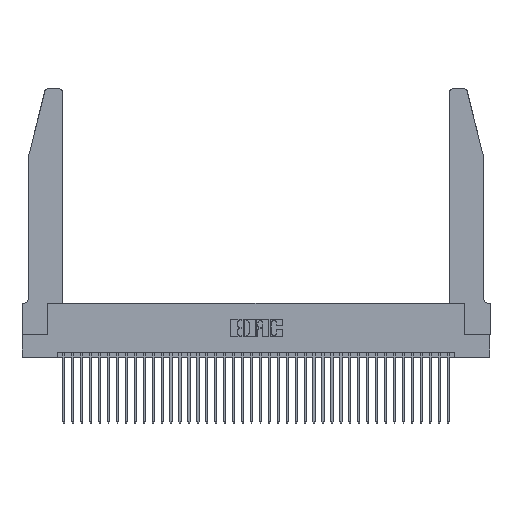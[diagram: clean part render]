
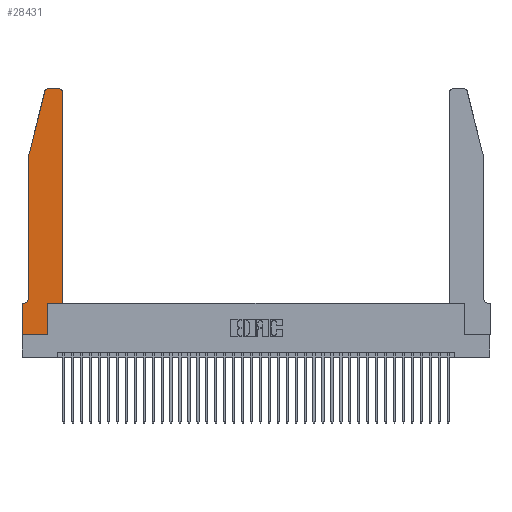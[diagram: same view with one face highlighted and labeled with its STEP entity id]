
A CAD part, top view. The second image highlights one B-rep face of the part: STEP entity #28431.
In plain terms, the highlighted planar face has unit normal (0, 0, 1).
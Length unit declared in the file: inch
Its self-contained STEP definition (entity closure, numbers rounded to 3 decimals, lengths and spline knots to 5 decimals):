
#224 = EDGE_CURVE ( 'NONE', #29891, #2892, #13376, .T. ) ;
#667 = CARTESIAN_POINT ( 'NONE',  ( 0.4505, 0.35, 0.37 ) ) ;
#727 = LINE ( 'NONE', #18603, #18625 ) ;
#1200 = VECTOR ( 'NONE', #37768, 39.37008 ) ;
#1596 = PLANE ( 'NONE',  #32120 ) ;
#1674 = ORIENTED_EDGE ( 'NONE', *, *, #16452, .T. ) ;
#2068 = DIRECTION ( 'NONE',  ( 1., 0., 0. ) ) ;
#2127 = VECTOR ( 'NONE', #15969, 39.37008 ) ;
#2576 = LINE ( 'NONE', #667, #2127 ) ;
#2687 = DIRECTION ( 'NONE',  ( -1., 0., 0. ) ) ;
#2892 = VERTEX_POINT ( 'NONE', #20717 ) ;
#4173 = VERTEX_POINT ( 'NONE', #35448 ) ;
#4774 = CARTESIAN_POINT ( 'NONE',  ( 0.2865, 0., 0.37 ) ) ;
#5202 = EDGE_CURVE ( 'NONE', #22852, #8527, #727, .T. ) ;
#5338 = CARTESIAN_POINT ( 'NONE',  ( 0.4505, 0.35, 0.37 ) ) ;
#5971 = CARTESIAN_POINT ( 'NONE',  ( 0., 0., 0.37 ) ) ;
#6291 = CARTESIAN_POINT ( 'NONE',  ( 0.284, 2.72, 0.37 ) ) ;
#6340 = ORIENTED_EDGE ( 'NONE', *, *, #35935, .T. ) ;
#6474 = ORIENTED_EDGE ( 'NONE', *, *, #19601, .T. ) ;
#7373 = FACE_OUTER_BOUND ( 'NONE', #20908, .T. ) ;
#7486 = VERTEX_POINT ( 'NONE', #33613 ) ;
#7542 = VECTOR ( 'NONE', #30701, 39.37008 ) ;
#7683 = ORIENTED_EDGE ( 'NONE', *, *, #36097, .T. ) ;
#8160 = VECTOR ( 'NONE', #17964, 39.37008 ) ;
#8347 = ORIENTED_EDGE ( 'NONE', *, *, #224, .T. ) ;
#8405 = VERTEX_POINT ( 'NONE', #4774 ) ;
#8527 = VERTEX_POINT ( 'NONE', #29966 ) ;
#9138 = CARTESIAN_POINT ( 'NONE',  ( 0.4505, 2.72, 0.37 ) ) ;
#9248 = ORIENTED_EDGE ( 'NONE', *, *, #34002, .T. ) ;
#10431 = VERTEX_POINT ( 'NONE', #27357 ) ;
#10446 = DIRECTION ( 'NONE',  ( 1., 0., 0. ) ) ;
#10654 = ORIENTED_EDGE ( 'NONE', *, *, #5202, .T. ) ;
#13376 = LINE ( 'NONE', #5971, #8160 ) ;
#14517 = EDGE_CURVE ( 'NONE', #10431, #18430, #16909, .T. ) ;
#15095 = LINE ( 'NONE', #36754, #7542 ) ;
#15705 = VECTOR ( 'NONE', #23273, 39.37008 ) ;
#15969 = DIRECTION ( 'NONE',  ( 0., 1., 0. ) ) ;
#16210 = ORIENTED_EDGE ( 'NONE', *, *, #38175, .T. ) ;
#16410 = ORIENTED_EDGE ( 'NONE', *, *, #17828, .T. ) ;
#16452 = EDGE_CURVE ( 'NONE', #2892, #8405, #31393, .T. ) ;
#16646 = LINE ( 'NONE', #16975, #15705 ) ;
#16909 = LINE ( 'NONE', #21971, #36721 ) ;
#16975 = CARTESIAN_POINT ( 'NONE',  ( 0.4505, 0.35, 0.37 ) ) ;
#17558 = EDGE_CURVE ( 'NONE', #18430, #4173, #30797, .T. ) ;
#17794 = LINE ( 'NONE', #25690, #23898 ) ;
#17828 = EDGE_CURVE ( 'NONE', #7486, #22150, #16646, .T. ) ;
#17964 = DIRECTION ( 'NONE',  ( 0., -1., 0. ) ) ;
#18154 = DIRECTION ( 'NONE',  ( 1., 0., 0. ) ) ;
#18430 = VERTEX_POINT ( 'NONE', #21197 ) ;
#18603 = CARTESIAN_POINT ( 'NONE',  ( 0.2605, 2.75, 0.37 ) ) ;
#18625 = VECTOR ( 'NONE', #21612, 39.37008 ) ;
#19601 = EDGE_CURVE ( 'NONE', #4173, #22254, #33695, .T. ) ;
#20607 = CARTESIAN_POINT ( 'NONE',  ( 0.0055, 0.42, 0.37 ) ) ;
#20717 = CARTESIAN_POINT ( 'NONE',  ( 0., 0., 0.37 ) ) ;
#20908 = EDGE_LOOP ( 'NONE', ( #10654, #6340, #33339, #28059, #6474, #20993, #8347, #1674, #7683, #16410, #9248, #16210 ) ) ;
#20993 = ORIENTED_EDGE ( 'NONE', *, *, #35702, .T. ) ;
#21197 = CARTESIAN_POINT ( 'NONE',  ( 0.0755, 2., 0.37 ) ) ;
#21612 = DIRECTION ( 'NONE',  ( -1., 0., 0. ) ) ;
#21971 = CARTESIAN_POINT ( 'NONE',  ( 0.0755, 2., 0.37 ) ) ;
#22077 = CARTESIAN_POINT ( 'NONE',  ( 0.0755, 2., 0.37 ) ) ;
#22150 = VERTEX_POINT ( 'NONE', #5338 ) ;
#22254 = VERTEX_POINT ( 'NONE', #30280 ) ;
#22585 = CARTESIAN_POINT ( 'NONE',  ( 0., 0., 0.37 ) ) ;
#22828 = CARTESIAN_POINT ( 'NONE',  ( 0., 0.35, 0.37 ) ) ;
#22852 = VERTEX_POINT ( 'NONE', #29315 ) ;
#23273 = DIRECTION ( 'NONE',  ( 1., 0., 0. ) ) ;
#23898 = VECTOR ( 'NONE', #28742, 39.37008 ) ;
#24985 = DIRECTION ( 'NONE',  ( 0., -1., 0. ) ) ;
#25690 = CARTESIAN_POINT ( 'NONE',  ( 0.0755, 0.35, 0.37 ) ) ;
#26410 = CIRCLE ( 'NONE', #27653, 0.03 ) ;
#26876 = VERTEX_POINT ( 'NONE', #9138 ) ;
#27357 = CARTESIAN_POINT ( 'NONE',  ( 0.25487, 2.72718, 0.37 ) ) ;
#27653 = AXIS2_PLACEMENT_3D ( 'NONE', #6291, #33208, #18154 ) ;
#27711 = AXIS2_PLACEMENT_3D ( 'NONE', #37686, #38213, #2068 ) ;
#28059 = ORIENTED_EDGE ( 'NONE', *, *, #17558, .T. ) ;
#28195 = DIRECTION ( 'NONE',  ( -0.239, -0.971, 0. ) ) ;
#28431 = ADVANCED_FACE ( 'NONE', ( #7373 ), #1596, .T. ) ;
#28493 = DIRECTION ( 'NONE',  ( 0., 0., 1. ) ) ;
#28742 = DIRECTION ( 'NONE',  ( -1., 0., 0. ) ) ;
#29315 = CARTESIAN_POINT ( 'NONE',  ( 0.4205, 2.75, 0.37 ) ) ;
#29629 = CIRCLE ( 'NONE', #27711, 0.03 ) ;
#29891 = VERTEX_POINT ( 'NONE', #22828 ) ;
#29966 = CARTESIAN_POINT ( 'NONE',  ( 0.284, 2.75, 0.37 ) ) ;
#30280 = CARTESIAN_POINT ( 'NONE',  ( 0.0055, 0.35, 0.37 ) ) ;
#30701 = DIRECTION ( 'NONE',  ( 0., 1., 0. ) ) ;
#30797 = LINE ( 'NONE', #22077, #38807 ) ;
#31393 = LINE ( 'NONE', #22585, #1200 ) ;
#32120 = AXIS2_PLACEMENT_3D ( 'NONE', #37730, #28493, #10446 ) ;
#33208 = DIRECTION ( 'NONE',  ( 0., 0., 1. ) ) ;
#33339 = ORIENTED_EDGE ( 'NONE', *, *, #14517, .T. ) ;
#33613 = CARTESIAN_POINT ( 'NONE',  ( 0.2865, 0.35, 0.37 ) ) ;
#33695 = CIRCLE ( 'NONE', #37466, 0.07 ) ;
#34002 = EDGE_CURVE ( 'NONE', #22150, #26876, #2576, .T. ) ;
#35448 = CARTESIAN_POINT ( 'NONE',  ( 0.0755, 0.42, 0.37 ) ) ;
#35702 = EDGE_CURVE ( 'NONE', #22254, #29891, #17794, .T. ) ;
#35824 = DIRECTION ( 'NONE',  ( 0., 0., -1. ) ) ;
#35935 = EDGE_CURVE ( 'NONE', #8527, #10431, #26410, .T. ) ;
#36097 = EDGE_CURVE ( 'NONE', #8405, #7486, #15095, .T. ) ;
#36721 = VECTOR ( 'NONE', #28195, 39.37008 ) ;
#36754 = CARTESIAN_POINT ( 'NONE',  ( 0.2865, 0.35, 0.37 ) ) ;
#37466 = AXIS2_PLACEMENT_3D ( 'NONE', #20607, #35824, #2687 ) ;
#37686 = CARTESIAN_POINT ( 'NONE',  ( 0.4205, 2.72, 0.37 ) ) ;
#37730 = CARTESIAN_POINT ( 'NONE',  ( 0., 0.35, 0.37 ) ) ;
#37768 = DIRECTION ( 'NONE',  ( 1., 0., 0. ) ) ;
#38175 = EDGE_CURVE ( 'NONE', #26876, #22852, #29629, .T. ) ;
#38213 = DIRECTION ( 'NONE',  ( 0., 0., 1. ) ) ;
#38807 = VECTOR ( 'NONE', #24985, 39.37008 ) ;
